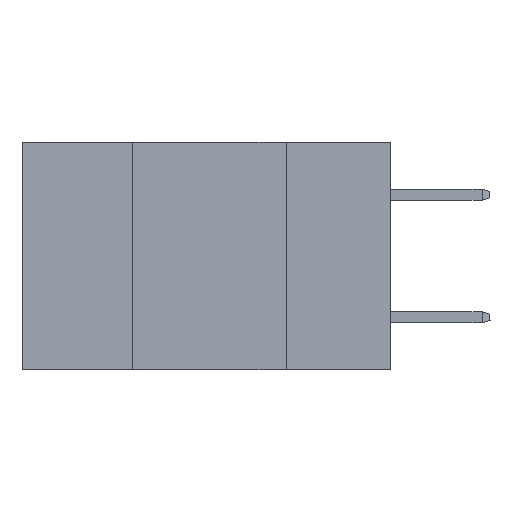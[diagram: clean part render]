
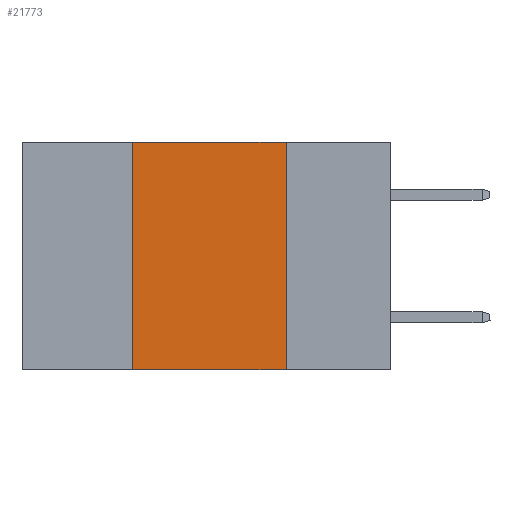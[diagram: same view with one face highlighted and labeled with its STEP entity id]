
A CAD part, left-side view. The second image highlights one B-rep face of the part: STEP entity #21773.
In plain terms, the highlighted planar face has unit normal (-1, 0, 0).
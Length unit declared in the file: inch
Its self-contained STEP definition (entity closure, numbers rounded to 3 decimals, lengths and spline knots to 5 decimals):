
#130 = VERTEX_POINT ( 'NONE', #29138 ) ;
#182 = CARTESIAN_POINT ( 'NONE',  ( 0., 0.17, 0. ) ) ;
#1476 = CARTESIAN_POINT ( 'NONE',  ( 0., 0.42, 0. ) ) ;
#1958 = EDGE_CURVE ( 'NONE', #130, #37960, #30773, .T. ) ;
#2091 = CARTESIAN_POINT ( 'NONE',  ( 0., 0.17, -0.37 ) ) ;
#3662 = VERTEX_POINT ( 'NONE', #11358 ) ;
#6652 = CARTESIAN_POINT ( 'NONE',  ( 0., 0.6, 0. ) ) ;
#6858 = DIRECTION ( 'NONE',  ( 1., 0., 0. ) ) ;
#8999 = LINE ( 'NONE', #182, #16237 ) ;
#10054 = DIRECTION ( 'NONE',  ( 0., 0., -1. ) ) ;
#10480 = CARTESIAN_POINT ( 'NONE',  ( 0., 0.6, -0.37 ) ) ;
#10938 = LINE ( 'NONE', #22538, #22066 ) ;
#11358 = CARTESIAN_POINT ( 'NONE',  ( 0., 0.17, 0. ) ) ;
#12106 = EDGE_CURVE ( 'NONE', #3662, #21561, #8999, .T. ) ;
#12657 = FACE_OUTER_BOUND ( 'NONE', #30649, .T. ) ;
#12904 = ORIENTED_EDGE ( 'NONE', *, *, #25066, .F. ) ;
#13143 = DIRECTION ( 'NONE',  ( 0., -1., 0. ) ) ;
#15599 = DIRECTION ( 'NONE',  ( 0., 0., 1. ) ) ;
#16237 = VECTOR ( 'NONE', #24977, 39.37008 ) ;
#21202 = ORIENTED_EDGE ( 'NONE', *, *, #12106, .F. ) ;
#21561 = VERTEX_POINT ( 'NONE', #2091 ) ;
#21773 = ADVANCED_FACE ( 'NONE', ( #12657 ), #28032, .F. ) ;
#21793 = CARTESIAN_POINT ( 'NONE',  ( 0., 0.42, 0. ) ) ;
#21884 = ORIENTED_EDGE ( 'NONE', *, *, #37946, .T. ) ;
#22066 = VECTOR ( 'NONE', #13143, 39.37008 ) ;
#22490 = LINE ( 'NONE', #10480, #31093 ) ;
#22538 = CARTESIAN_POINT ( 'NONE',  ( 0., 0.6, 0. ) ) ;
#22680 = DIRECTION ( 'NONE',  ( 0., -1., 0. ) ) ;
#24977 = DIRECTION ( 'NONE',  ( 0., 0., -1. ) ) ;
#25066 = EDGE_CURVE ( 'NONE', #37960, #3662, #10938, .T. ) ;
#28032 = PLANE ( 'NONE',  #35269 ) ;
#29138 = CARTESIAN_POINT ( 'NONE',  ( 0., 0.42, -0.37 ) ) ;
#30649 = EDGE_LOOP ( 'NONE', ( #21202, #12904, #38779, #21884 ) ) ;
#30773 = LINE ( 'NONE', #21793, #35721 ) ;
#31093 = VECTOR ( 'NONE', #22680, 39.37008 ) ;
#35269 = AXIS2_PLACEMENT_3D ( 'NONE', #6652, #6858, #10054 ) ;
#35721 = VECTOR ( 'NONE', #15599, 39.37008 ) ;
#37946 = EDGE_CURVE ( 'NONE', #130, #21561, #22490, .T. ) ;
#37960 = VERTEX_POINT ( 'NONE', #1476 ) ;
#38779 = ORIENTED_EDGE ( 'NONE', *, *, #1958, .F. ) ;
